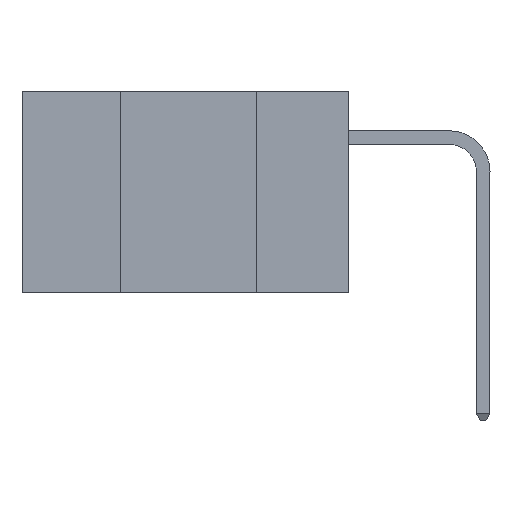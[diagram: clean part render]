
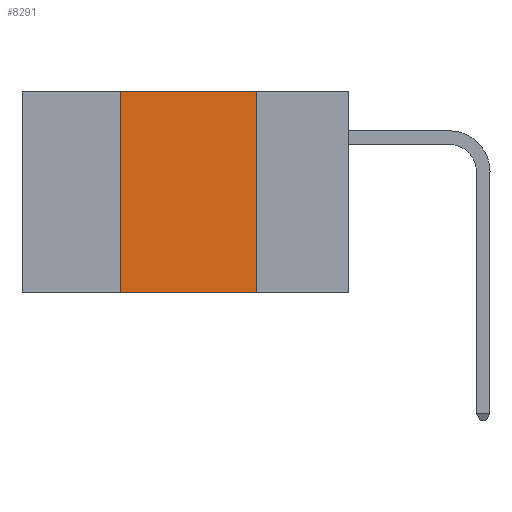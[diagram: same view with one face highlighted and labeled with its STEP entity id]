
A CAD part, left-side view. The second image highlights one B-rep face of the part: STEP entity #8291.
In plain terms, the highlighted planar face has unit normal (-1, 0, 0).
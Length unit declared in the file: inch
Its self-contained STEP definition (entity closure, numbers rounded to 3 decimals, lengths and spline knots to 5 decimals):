
#582 = CARTESIAN_POINT ( 'NONE',  ( 0., 0.42, 0. ) ) ;
#597 = EDGE_CURVE ( 'NONE', #1403, #8982, #5566, .T. ) ;
#961 = ORIENTED_EDGE ( 'NONE', *, *, #4446, .F. ) ;
#1403 = VERTEX_POINT ( 'NONE', #11225 ) ;
#1609 = PLANE ( 'NONE',  #5300 ) ;
#2117 = VERTEX_POINT ( 'NONE', #582 ) ;
#2497 = DIRECTION ( 'NONE',  ( 1., 0., 0. ) ) ;
#2533 = EDGE_CURVE ( 'NONE', #8819, #8982, #11071, .T. ) ;
#2598 = DIRECTION ( 'NONE',  ( 0., -1., 0. ) ) ;
#2736 = CARTESIAN_POINT ( 'NONE',  ( 0., 0.17, 0. ) ) ;
#3403 = VECTOR ( 'NONE', #10965, 39.37008 ) ;
#3798 = FACE_OUTER_BOUND ( 'NONE', #9347, .T. ) ;
#3916 = LINE ( 'NONE', #7074, #6004 ) ;
#4184 = DIRECTION ( 'NONE',  ( 0., 0., -1. ) ) ;
#4446 = EDGE_CURVE ( 'NONE', #8819, #2117, #5789, .T. ) ;
#5156 = ORIENTED_EDGE ( 'NONE', *, *, #9068, .F. ) ;
#5224 = CARTESIAN_POINT ( 'NONE',  ( 0., 0.17, -0.37 ) ) ;
#5300 = AXIS2_PLACEMENT_3D ( 'NONE', #7853, #2497, #8705 ) ;
#5566 = LINE ( 'NONE', #2736, #7674 ) ;
#5789 = LINE ( 'NONE', #10139, #3403 ) ;
#6004 = VECTOR ( 'NONE', #2598, 39.37008 ) ;
#7074 = CARTESIAN_POINT ( 'NONE',  ( 0., 0.6, 0. ) ) ;
#7482 = CARTESIAN_POINT ( 'NONE',  ( 0., 0.6, -0.37 ) ) ;
#7674 = VECTOR ( 'NONE', #4184, 39.37008 ) ;
#7853 = CARTESIAN_POINT ( 'NONE',  ( 0., 0.6, 0. ) ) ;
#8078 = ORIENTED_EDGE ( 'NONE', *, *, #2533, .T. ) ;
#8291 = ADVANCED_FACE ( 'NONE', ( #3798 ), #1609, .F. ) ;
#8705 = DIRECTION ( 'NONE',  ( 0., 0., -1. ) ) ;
#8819 = VERTEX_POINT ( 'NONE', #11037 ) ;
#8982 = VERTEX_POINT ( 'NONE', #5224 ) ;
#9068 = EDGE_CURVE ( 'NONE', #2117, #1403, #3916, .T. ) ;
#9347 = EDGE_LOOP ( 'NONE', ( #9463, #5156, #961, #8078 ) ) ;
#9463 = ORIENTED_EDGE ( 'NONE', *, *, #597, .F. ) ;
#10139 = CARTESIAN_POINT ( 'NONE',  ( 0., 0.42, 0. ) ) ;
#10802 = VECTOR ( 'NONE', #10884, 39.37008 ) ;
#10884 = DIRECTION ( 'NONE',  ( 0., -1., 0. ) ) ;
#10965 = DIRECTION ( 'NONE',  ( 0., 0., 1. ) ) ;
#11037 = CARTESIAN_POINT ( 'NONE',  ( 0., 0.42, -0.37 ) ) ;
#11071 = LINE ( 'NONE', #7482, #10802 ) ;
#11225 = CARTESIAN_POINT ( 'NONE',  ( 0., 0.17, 0. ) ) ;
